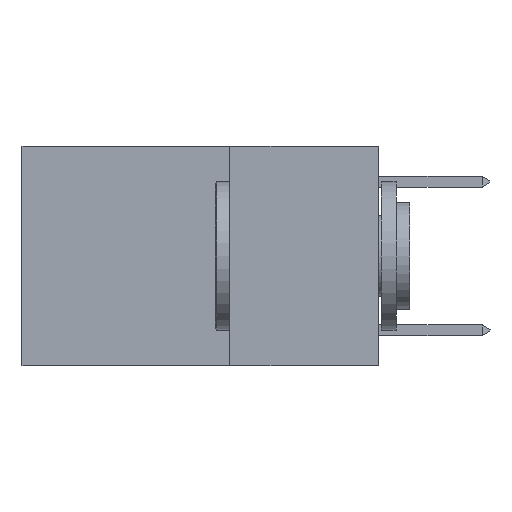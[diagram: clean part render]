
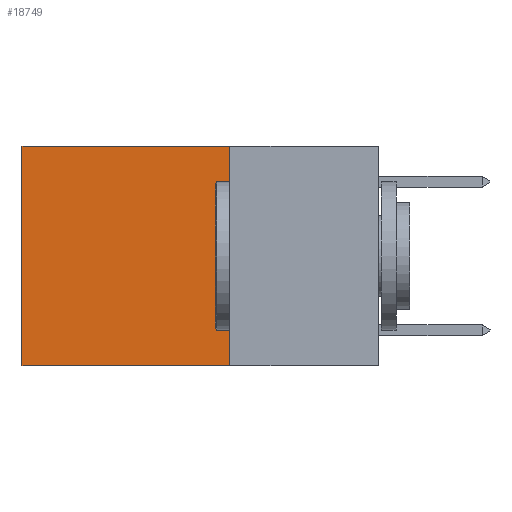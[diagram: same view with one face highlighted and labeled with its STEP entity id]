
A CAD part, left-side view. The second image highlights one B-rep face of the part: STEP entity #18749.
In plain terms, the highlighted planar face has unit normal (-1, 0, 0).
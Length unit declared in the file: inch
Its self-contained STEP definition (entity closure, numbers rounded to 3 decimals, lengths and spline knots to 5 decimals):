
#254 = CARTESIAN_POINT ( 'NONE',  ( 0.2625, 0.6, 0. ) ) ;
#1452 = ORIENTED_EDGE ( 'NONE', *, *, #21394, .T. ) ;
#1764 = LINE ( 'NONE', #254, #1963 ) ;
#1963 = VECTOR ( 'NONE', #12766, 39.37008 ) ;
#2568 = ORIENTED_EDGE ( 'NONE', *, *, #16157, .T. ) ;
#2995 = DIRECTION ( 'NONE',  ( 0., 0., -1. ) ) ;
#5587 = PLANE ( 'NONE',  #15592 ) ;
#5779 = ORIENTED_EDGE ( 'NONE', *, *, #10408, .F. ) ;
#6275 = CARTESIAN_POINT ( 'NONE',  ( 0.2625, 0.25, -0.37 ) ) ;
#6604 = VECTOR ( 'NONE', #6804, 39.37008 ) ;
#6612 = LINE ( 'NONE', #7507, #6604 ) ;
#6804 = DIRECTION ( 'NONE',  ( 0., 1., 0. ) ) ;
#7113 = CARTESIAN_POINT ( 'NONE',  ( 0.2625, 0.6, 0. ) ) ;
#7507 = CARTESIAN_POINT ( 'NONE',  ( 0.2625, 0.25, -0.37 ) ) ;
#7722 = VERTEX_POINT ( 'NONE', #6275 ) ;
#8120 = CARTESIAN_POINT ( 'NONE',  ( 0.2625, 0.25, 0. ) ) ;
#8625 = EDGE_CURVE ( 'NONE', #7722, #12970, #6612, .T. ) ;
#8946 = EDGE_LOOP ( 'NONE', ( #1452, #14856, #5779, #2568 ) ) ;
#9175 = CARTESIAN_POINT ( 'NONE',  ( 0.2625, 0.25, 0. ) ) ;
#10408 = EDGE_CURVE ( 'NONE', #10540, #7722, #19755, .T. ) ;
#10540 = VERTEX_POINT ( 'NONE', #17208 ) ;
#10975 = DIRECTION ( 'NONE',  ( 0., 0., -1. ) ) ;
#11675 = DIRECTION ( 'NONE',  ( 0., 1., 0. ) ) ;
#12766 = DIRECTION ( 'NONE',  ( 0., 0., -1. ) ) ;
#12970 = VERTEX_POINT ( 'NONE', #16955 ) ;
#13049 = VECTOR ( 'NONE', #11675, 39.37008 ) ;
#13265 = LINE ( 'NONE', #8120, #13049 ) ;
#14856 = ORIENTED_EDGE ( 'NONE', *, *, #8625, .F. ) ;
#14973 = VERTEX_POINT ( 'NONE', #7113 ) ;
#15592 = AXIS2_PLACEMENT_3D ( 'NONE', #9175, #20702, #10975 ) ;
#16157 = EDGE_CURVE ( 'NONE', #10540, #14973, #13265, .T. ) ;
#16955 = CARTESIAN_POINT ( 'NONE',  ( 0.2625, 0.6, -0.37 ) ) ;
#17208 = CARTESIAN_POINT ( 'NONE',  ( 0.2625, 0.25, 0. ) ) ;
#18212 = FACE_OUTER_BOUND ( 'NONE', #8946, .T. ) ;
#18749 = ADVANCED_FACE ( 'NONE', ( #18212 ), #5587, .F. ) ;
#19692 = VECTOR ( 'NONE', #2995, 39.37008 ) ;
#19755 = LINE ( 'NONE', #21497, #19692 ) ;
#20702 = DIRECTION ( 'NONE',  ( 1., 0., 0. ) ) ;
#21394 = EDGE_CURVE ( 'NONE', #14973, #12970, #1764, .T. ) ;
#21497 = CARTESIAN_POINT ( 'NONE',  ( 0.2625, 0.25, 0. ) ) ;
